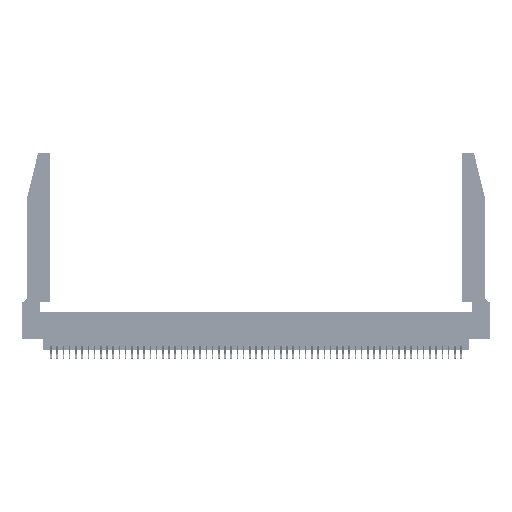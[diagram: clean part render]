
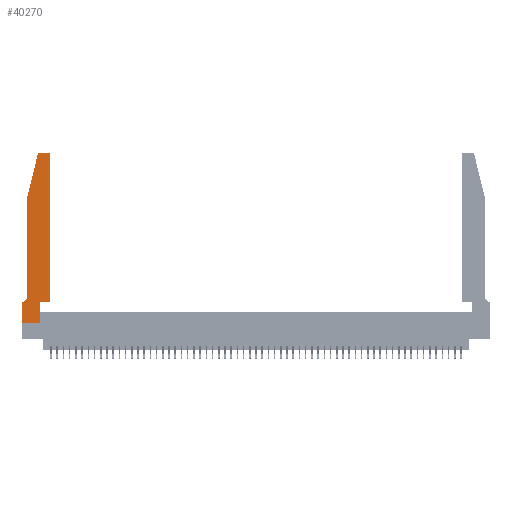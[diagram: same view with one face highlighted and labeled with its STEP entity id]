
A CAD part, top view. The second image highlights one B-rep face of the part: STEP entity #40270.
In plain terms, the highlighted planar face has unit normal (0, 0, 1).
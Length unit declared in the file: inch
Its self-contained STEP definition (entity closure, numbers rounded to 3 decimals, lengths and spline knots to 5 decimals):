
#338 = VERTEX_POINT ( 'NONE', #2395 ) ;
#1376 = VECTOR ( 'NONE', #31445, 39.37008 ) ;
#1518 = VECTOR ( 'NONE', #30849, 39.37008 ) ;
#2395 = CARTESIAN_POINT ( 'NONE',  ( 0.4505, 0.35, 0.37 ) ) ;
#2459 = CARTESIAN_POINT ( 'NONE',  ( 0.0755, 2., 0.37 ) ) ;
#3814 = CARTESIAN_POINT ( 'NONE',  ( 0., 0.35, 0.37 ) ) ;
#4050 = LINE ( 'NONE', #10357, #1376 ) ;
#4685 = ORIENTED_EDGE ( 'NONE', *, *, #5123, .T. ) ;
#4951 = ORIENTED_EDGE ( 'NONE', *, *, #34903, .T. ) ;
#5123 = EDGE_CURVE ( 'NONE', #10707, #40409, #28830, .T. ) ;
#5492 = ORIENTED_EDGE ( 'NONE', *, *, #20600, .T. ) ;
#5719 = LINE ( 'NONE', #21704, #30648 ) ;
#6851 = DIRECTION ( 'NONE',  ( -0.239, -0.971, 0. ) ) ;
#7453 = AXIS2_PLACEMENT_3D ( 'NONE', #46304, #45755, #8167 ) ;
#8118 = CARTESIAN_POINT ( 'NONE',  ( 0.2605, 2.75, 0.37 ) ) ;
#8167 = DIRECTION ( 'NONE',  ( 1., 0., 0. ) ) ;
#8194 = DIRECTION ( 'NONE',  ( 1., 0., 0. ) ) ;
#8764 = CARTESIAN_POINT ( 'NONE',  ( 0., 0., 0.37 ) ) ;
#10214 = EDGE_CURVE ( 'NONE', #25982, #10707, #45910, .T. ) ;
#10357 = CARTESIAN_POINT ( 'NONE',  ( 0.0755, 2., 0.37 ) ) ;
#10429 = VECTOR ( 'NONE', #16130, 39.37008 ) ;
#10707 = VERTEX_POINT ( 'NONE', #42078 ) ;
#10987 = DIRECTION ( 'NONE',  ( 0., 1., 0. ) ) ;
#11839 = AXIS2_PLACEMENT_3D ( 'NONE', #29452, #33511, #24470 ) ;
#14672 = EDGE_CURVE ( 'NONE', #30552, #43361, #20446, .T. ) ;
#15259 = LINE ( 'NONE', #2459, #54013 ) ;
#15288 = AXIS2_PLACEMENT_3D ( 'NONE', #3814, #16788, #46155 ) ;
#16101 = VECTOR ( 'NONE', #10987, 39.37008 ) ;
#16130 = DIRECTION ( 'NONE',  ( 1., 0., 0. ) ) ;
#16504 = CARTESIAN_POINT ( 'NONE',  ( 0.2865, 0.35, 0.37 ) ) ;
#16788 = DIRECTION ( 'NONE',  ( 0., 0., 1. ) ) ;
#16800 = EDGE_CURVE ( 'NONE', #43361, #38444, #5719, .T. ) ;
#17100 = ORIENTED_EDGE ( 'NONE', *, *, #10214, .T. ) ;
#17262 = CARTESIAN_POINT ( 'NONE',  ( 0.2865, 0.35, 0.37 ) ) ;
#17344 = CARTESIAN_POINT ( 'NONE',  ( 0.0055, 0.35, 0.37 ) ) ;
#17785 = EDGE_CURVE ( 'NONE', #338, #25982, #27908, .T. ) ;
#17829 = CARTESIAN_POINT ( 'NONE',  ( 0.25487, 2.72718, 0.37 ) ) ;
#17994 = ORIENTED_EDGE ( 'NONE', *, *, #32229, .T. ) ;
#18030 = DIRECTION ( 'NONE',  ( 0., -1., 0. ) ) ;
#18380 = CARTESIAN_POINT ( 'NONE',  ( 0.0755, 0.35, 0.37 ) ) ;
#19151 = VERTEX_POINT ( 'NONE', #26844 ) ;
#19283 = CARTESIAN_POINT ( 'NONE',  ( 0., 0.35, 0.37 ) ) ;
#19577 = CIRCLE ( 'NONE', #28259, 0.07 ) ;
#20446 = LINE ( 'NONE', #18380, #1518 ) ;
#20600 = EDGE_CURVE ( 'NONE', #19151, #40053, #4050, .T. ) ;
#21562 = CARTESIAN_POINT ( 'NONE',  ( 0.284, 2.75, 0.37 ) ) ;
#21593 = ORIENTED_EDGE ( 'NONE', *, *, #39557, .T. ) ;
#21704 = CARTESIAN_POINT ( 'NONE',  ( 0., 0., 0.37 ) ) ;
#24470 = DIRECTION ( 'NONE',  ( 1., 0., 0. ) ) ;
#25472 = DIRECTION ( 'NONE',  ( -1., 0., 0. ) ) ;
#25474 = DIRECTION ( 'NONE',  ( 0., 1., 0. ) ) ;
#25727 = ORIENTED_EDGE ( 'NONE', *, *, #14672, .T. ) ;
#25738 = ORIENTED_EDGE ( 'NONE', *, *, #16800, .T. ) ;
#25742 = LINE ( 'NONE', #17262, #29068 ) ;
#25928 = VERTEX_POINT ( 'NONE', #30313 ) ;
#25982 = VERTEX_POINT ( 'NONE', #29203 ) ;
#26289 = ORIENTED_EDGE ( 'NONE', *, *, #51121, .T. ) ;
#26844 = CARTESIAN_POINT ( 'NONE',  ( 0.0755, 2., 0.37 ) ) ;
#27514 = VECTOR ( 'NONE', #25472, 39.37008 ) ;
#27765 = LINE ( 'NONE', #50558, #39614 ) ;
#27908 = LINE ( 'NONE', #27980, #16101 ) ;
#27980 = CARTESIAN_POINT ( 'NONE',  ( 0.4505, 0.35, 0.37 ) ) ;
#28077 = VERTEX_POINT ( 'NONE', #17829 ) ;
#28259 = AXIS2_PLACEMENT_3D ( 'NONE', #52638, #44346, #31705 ) ;
#28830 = LINE ( 'NONE', #8118, #27514 ) ;
#29068 = VECTOR ( 'NONE', #25474, 39.37008 ) ;
#29203 = CARTESIAN_POINT ( 'NONE',  ( 0.4505, 2.72, 0.37 ) ) ;
#29452 = CARTESIAN_POINT ( 'NONE',  ( 0.4205, 2.72, 0.37 ) ) ;
#30102 = LINE ( 'NONE', #37060, #10429 ) ;
#30313 = CARTESIAN_POINT ( 'NONE',  ( 0.2865, 0., 0.37 ) ) ;
#30552 = VERTEX_POINT ( 'NONE', #17344 ) ;
#30648 = VECTOR ( 'NONE', #18030, 39.37008 ) ;
#30849 = DIRECTION ( 'NONE',  ( -1., 0., 0. ) ) ;
#31244 = EDGE_LOOP ( 'NONE', ( #4685, #4951, #17994, #5492, #40403, #25727, #25738, #21593, #38314, #26289, #50966, #17100 ) ) ;
#31445 = DIRECTION ( 'NONE',  ( 0., -1., 0. ) ) ;
#31705 = DIRECTION ( 'NONE',  ( -1., 0., 0. ) ) ;
#32229 = EDGE_CURVE ( 'NONE', #28077, #19151, #15259, .T. ) ;
#33511 = DIRECTION ( 'NONE',  ( 0., 0., 1. ) ) ;
#34903 = EDGE_CURVE ( 'NONE', #40409, #28077, #52403, .T. ) ;
#37060 = CARTESIAN_POINT ( 'NONE',  ( 0., 0., 0.37 ) ) ;
#37169 = EDGE_CURVE ( 'NONE', #25928, #43586, #25742, .T. ) ;
#38314 = ORIENTED_EDGE ( 'NONE', *, *, #37169, .T. ) ;
#38444 = VERTEX_POINT ( 'NONE', #8764 ) ;
#39557 = EDGE_CURVE ( 'NONE', #38444, #25928, #30102, .T. ) ;
#39614 = VECTOR ( 'NONE', #8194, 39.37008 ) ;
#39970 = EDGE_CURVE ( 'NONE', #40053, #30552, #19577, .T. ) ;
#40053 = VERTEX_POINT ( 'NONE', #53342 ) ;
#40270 = ADVANCED_FACE ( 'NONE', ( #40516 ), #41375, .T. ) ;
#40403 = ORIENTED_EDGE ( 'NONE', *, *, #39970, .T. ) ;
#40409 = VERTEX_POINT ( 'NONE', #21562 ) ;
#40516 = FACE_OUTER_BOUND ( 'NONE', #31244, .T. ) ;
#41375 = PLANE ( 'NONE',  #15288 ) ;
#42078 = CARTESIAN_POINT ( 'NONE',  ( 0.4205, 2.75, 0.37 ) ) ;
#43361 = VERTEX_POINT ( 'NONE', #19283 ) ;
#43586 = VERTEX_POINT ( 'NONE', #16504 ) ;
#44346 = DIRECTION ( 'NONE',  ( 0., 0., -1. ) ) ;
#45755 = DIRECTION ( 'NONE',  ( 0., 0., 1. ) ) ;
#45910 = CIRCLE ( 'NONE', #11839, 0.03 ) ;
#46155 = DIRECTION ( 'NONE',  ( 1., 0., 0. ) ) ;
#46304 = CARTESIAN_POINT ( 'NONE',  ( 0.284, 2.72, 0.37 ) ) ;
#50558 = CARTESIAN_POINT ( 'NONE',  ( 0.4505, 0.35, 0.37 ) ) ;
#50966 = ORIENTED_EDGE ( 'NONE', *, *, #17785, .T. ) ;
#51121 = EDGE_CURVE ( 'NONE', #43586, #338, #27765, .T. ) ;
#52403 = CIRCLE ( 'NONE', #7453, 0.03 ) ;
#52638 = CARTESIAN_POINT ( 'NONE',  ( 0.0055, 0.42, 0.37 ) ) ;
#53342 = CARTESIAN_POINT ( 'NONE',  ( 0.0755, 0.42, 0.37 ) ) ;
#54013 = VECTOR ( 'NONE', #6851, 39.37008 ) ;
